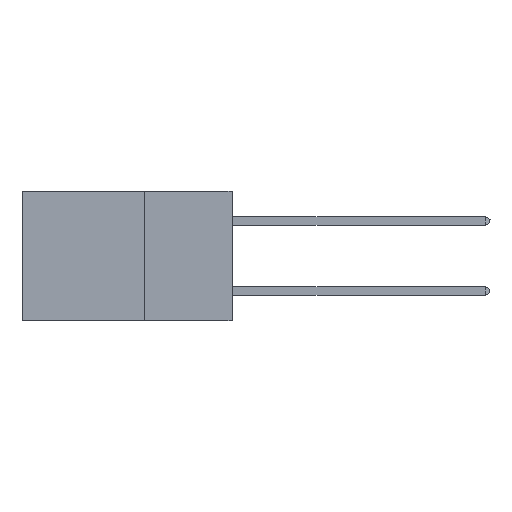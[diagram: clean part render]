
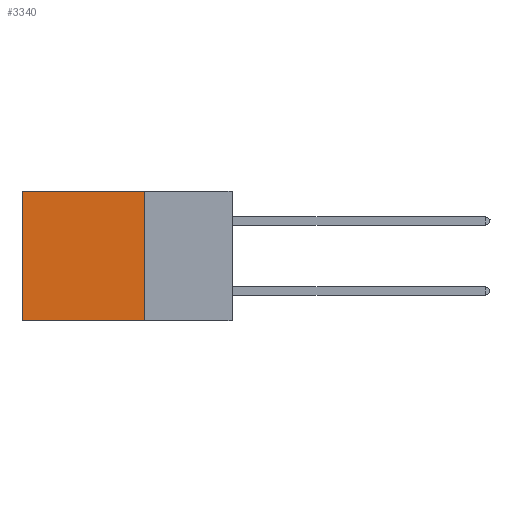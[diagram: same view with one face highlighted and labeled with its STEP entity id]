
A CAD part, left-side view. The second image highlights one B-rep face of the part: STEP entity #3340.
In plain terms, the highlighted planar face has unit normal (-1, 0, 0).
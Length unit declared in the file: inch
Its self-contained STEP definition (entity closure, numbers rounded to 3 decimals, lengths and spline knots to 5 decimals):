
#246 = LINE ( 'NONE', #5922, #19321 ) ;
#921 = EDGE_CURVE ( 'NONE', #1639, #17733, #14884, .T. ) ;
#1084 = EDGE_LOOP ( 'NONE', ( #14097, #2236, #20869, #22278 ) ) ;
#1639 = VERTEX_POINT ( 'NONE', #17760 ) ;
#2236 = ORIENTED_EDGE ( 'NONE', *, *, #23368, .F. ) ;
#3163 = EDGE_CURVE ( 'NONE', #1639, #16027, #11990, .T. ) ;
#3340 = ADVANCED_FACE ( 'NONE', ( #17585 ), #9330, .F. ) ;
#5079 = VECTOR ( 'NONE', #5796, 39.37008 ) ;
#5274 = AXIS2_PLACEMENT_3D ( 'NONE', #13060, #16653, #5715 ) ;
#5715 = DIRECTION ( 'NONE',  ( 0., 0., -1. ) ) ;
#5796 = DIRECTION ( 'NONE',  ( 0., 1., 0. ) ) ;
#5922 = CARTESIAN_POINT ( 'NONE',  ( 0.2875, 0.25, -0.37 ) ) ;
#6108 = CARTESIAN_POINT ( 'NONE',  ( 0.2875, 0.6, 0. ) ) ;
#7171 = CARTESIAN_POINT ( 'NONE',  ( 0.2875, 0.6, 0. ) ) ;
#7984 = DIRECTION ( 'NONE',  ( 0., 0., -1. ) ) ;
#9012 = CARTESIAN_POINT ( 'NONE',  ( 0.2875, 0.25, 0. ) ) ;
#9330 = PLANE ( 'NONE',  #5274 ) ;
#10481 = CARTESIAN_POINT ( 'NONE',  ( 0.2875, 0.6, -0.37 ) ) ;
#11266 = VECTOR ( 'NONE', #7984, 39.37008 ) ;
#11990 = LINE ( 'NONE', #9012, #16758 ) ;
#13060 = CARTESIAN_POINT ( 'NONE',  ( 0.2875, 0.25, 0. ) ) ;
#14097 = ORIENTED_EDGE ( 'NONE', *, *, #15506, .T. ) ;
#14884 = LINE ( 'NONE', #15686, #5079 ) ;
#15121 = DIRECTION ( 'NONE',  ( 0., 1., 0. ) ) ;
#15506 = EDGE_CURVE ( 'NONE', #17733, #21152, #20792, .T. ) ;
#15686 = CARTESIAN_POINT ( 'NONE',  ( 0.2875, 0.25, 0. ) ) ;
#16027 = VERTEX_POINT ( 'NONE', #21996 ) ;
#16653 = DIRECTION ( 'NONE',  ( 1., 0., 0. ) ) ;
#16758 = VECTOR ( 'NONE', #19786, 39.37008 ) ;
#17585 = FACE_OUTER_BOUND ( 'NONE', #1084, .T. ) ;
#17733 = VERTEX_POINT ( 'NONE', #7171 ) ;
#17760 = CARTESIAN_POINT ( 'NONE',  ( 0.2875, 0.25, 0. ) ) ;
#19321 = VECTOR ( 'NONE', #15121, 39.37008 ) ;
#19786 = DIRECTION ( 'NONE',  ( 0., 0., -1. ) ) ;
#20792 = LINE ( 'NONE', #6108, #11266 ) ;
#20869 = ORIENTED_EDGE ( 'NONE', *, *, #3163, .F. ) ;
#21152 = VERTEX_POINT ( 'NONE', #10481 ) ;
#21996 = CARTESIAN_POINT ( 'NONE',  ( 0.2875, 0.25, -0.37 ) ) ;
#22278 = ORIENTED_EDGE ( 'NONE', *, *, #921, .T. ) ;
#23368 = EDGE_CURVE ( 'NONE', #16027, #21152, #246, .T. ) ;
